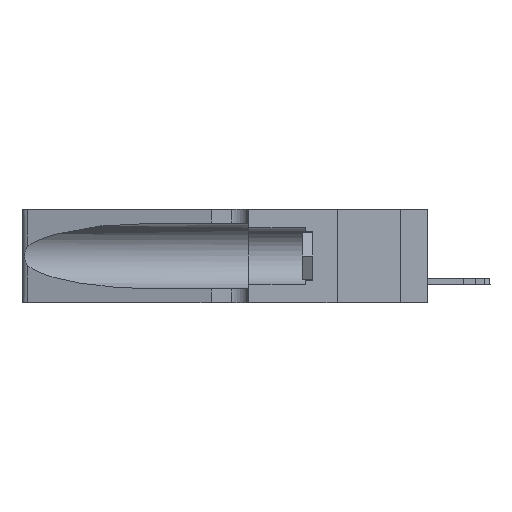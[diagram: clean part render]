
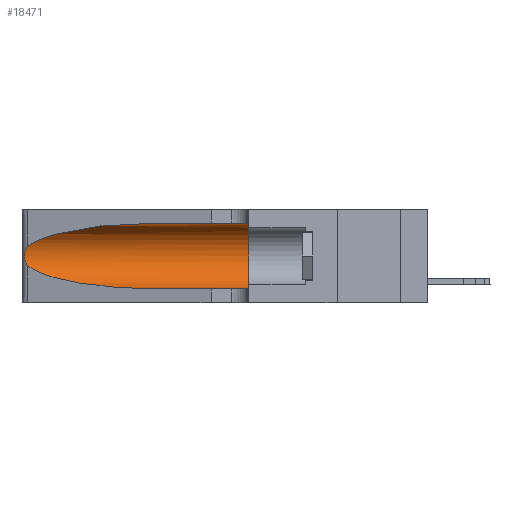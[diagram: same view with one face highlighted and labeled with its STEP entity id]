
A CAD part, left-side view. The second image highlights one B-rep face of the part: STEP entity #18471.
In plain terms, the highlighted cylindrical face has radius 3.308 mm (diameter 6.617 mm), a partial arc.
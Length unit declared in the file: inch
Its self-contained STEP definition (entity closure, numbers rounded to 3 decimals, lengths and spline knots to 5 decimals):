
#444 = CARTESIAN_POINT ( 'NONE',  ( 0.25555, 1.22993, 0.14849 ) ) ;
#629 = CARTESIAN_POINT ( 'NONE',  ( 0.25856, 1.23593, 0.16098 ) ) ;
#2391 = EDGE_CURVE ( 'NONE', #11627, #21126, #16305, .T. ) ;
#3287 = AXIS2_PLACEMENT_3D ( 'NONE', #11746, #11648, #22565 ) ;
#3627 = DIRECTION ( 'NONE',  ( 0., 1., 0. ) ) ;
#3782 = ORIENTED_EDGE ( 'NONE', *, *, #18995, .F. ) ;
#4146 = CARTESIAN_POINT ( 'NONE',  ( 0.1305, 1.61858, 0.31525 ) ) ;
#4651 = CARTESIAN_POINT ( 'NONE',  ( 0.26018, 1.23835, 0.19895 ) ) ;
#4823 = CARTESIAN_POINT ( 'NONE',  ( 0.25487, 1.22718, 0.22369 ) ) ;
#4932 = CARTESIAN_POINT ( 'NONE',  ( 0.25854, 1.2359, 0.20912 ) ) ;
#5532 = VERTEX_POINT ( 'NONE', #6572 ) ;
#6538 = CARTESIAN_POINT ( 'NONE',  ( 0.1305, 0.35, 0.05475 ) ) ;
#6572 = CARTESIAN_POINT ( 'NONE',  ( 0.1305, 0.35, 0.31525 ) ) ;
#6607 = CARTESIAN_POINT ( 'NONE',  ( 0.2373, 1.15595, 0.28018 ) ) ;
#6708 = CARTESIAN_POINT ( 'NONE',  ( 0.25639, 1.23184, 0.21858 ) ) ;
#6809 = CARTESIAN_POINT ( 'NONE',  ( 0.26075, 1.23896, 0.178 ) ) ;
#7101 = CARTESIAN_POINT ( 'NONE',  ( 0.26017, 1.23833, 0.17102 ) ) ;
#8749 = LINE ( 'NONE', #4146, #11160 ) ;
#9212 = CARTESIAN_POINT ( 'NONE',  ( 0.25487, 1.22718, 0.22369 ) ) ;
#9424 = VERTEX_POINT ( 'NONE', #26020 ) ;
#9692 = ORIENTED_EDGE ( 'NONE', *, *, #2391, .T. ) ;
#10090 = DIRECTION ( 'NONE',  ( 0., 0., 1. ) ) ;
#11160 = VECTOR ( 'NONE', #28088, 39.37008 ) ;
#11320 = CARTESIAN_POINT ( 'NONE',  ( 0.18966, 0.96281, 0.31525 ) ) ;
#11330 = CARTESIAN_POINT ( 'NONE',  ( 0.26075, 1.23896, 0.19203 ) ) ;
#11583 = CARTESIAN_POINT ( 'NONE',  ( 0.25487, 1.22718, 0.14631 ) ) ;
#11627 = VERTEX_POINT ( 'NONE', #17317 ) ;
#11648 = DIRECTION ( 'NONE',  ( 0., -1., 0. ) ) ;
#11746 = CARTESIAN_POINT ( 'NONE',  ( 0.1305, 1.61858, 0.185 ) ) ;
#11771 = CARTESIAN_POINT ( 'NONE',  ( 0.2373, 1.15595, 0.08982 ) ) ;
#12142 = VERTEX_POINT ( 'NONE', #22823 ) ;
#13289 = EDGE_LOOP ( 'NONE', ( #24638, #23947, #15255, #9692, #3782, #23756 ) ) ;
#13752 = EDGE_CURVE ( 'NONE', #9424, #12142, #21195, .T. ) ;
#13777 = CARTESIAN_POINT ( 'NONE',  ( 0.18966, 0.96281, 0.05475 ) ) ;
#14587 =( BOUNDED_CURVE ( )  B_SPLINE_CURVE ( 3, ( #11583, #11771, #13777, #18427 ),
 .UNSPECIFIED., .F., .F. ) 
 B_SPLINE_CURVE_WITH_KNOTS ( ( 4, 4 ),
 ( 3.44316, 4.71239 ),
 .UNSPECIFIED. ) 
 CURVE ( )  GEOMETRIC_REPRESENTATION_ITEM ( )  RATIONAL_B_SPLINE_CURVE ( ( 1., 0.87, 0.87, 1. ) ) 
 REPRESENTATION_ITEM ( '' )  );
#14685 = FACE_OUTER_BOUND ( 'NONE', #13289, .T. ) ;
#14928 = VECTOR ( 'NONE', #20136, 39.37008 ) ;
#15229 = CIRCLE ( 'NONE', #15394, 0.13025 ) ;
#15255 = ORIENTED_EDGE ( 'NONE', *, *, #19546, .T. ) ;
#15394 = AXIS2_PLACEMENT_3D ( 'NONE', #23144, #3627, #10090 ) ;
#16305 = LINE ( 'NONE', #24623, #14928 ) ;
#17317 = CARTESIAN_POINT ( 'NONE',  ( 0.1305, 0.72297, 0.05475 ) ) ;
#18016 = CARTESIAN_POINT ( 'NONE',  ( 0.25787, 1.23484, 0.2124 ) ) ;
#18427 = CARTESIAN_POINT ( 'NONE',  ( 0.1305, 0.72297, 0.05475 ) ) ;
#18471 = ADVANCED_FACE ( 'NONE', ( #14685 ), #21484, .F. ) ;
#18995 = EDGE_CURVE ( 'NONE', #5532, #21126, #15229, .T. ) ;
#19546 = EDGE_CURVE ( 'NONE', #12142, #11627, #14587, .T. ) ;
#19724 = CARTESIAN_POINT ( 'NONE',  ( 0.1305, 0.72297, 0.31525 ) ) ;
#20136 = DIRECTION ( 'NONE',  ( 0., -1., 0. ) ) ;
#21126 = VERTEX_POINT ( 'NONE', #6538 ) ;
#21195 = B_SPLINE_CURVE_WITH_KNOTS ( 'NONE', 3,
 ( #9212, #26789, #6708, #18016, #4932, #4651, #11330, #6809, #7101, #629, #21982, #22340, #444, #26680 ),
 .UNSPECIFIED., .F., .F.,
 ( 4, 2, 2, 2, 2, 2, 4 ),
 ( 0., 0.00027, 0.00053, 0.00107, 0.0016, 0.00187, 0.00214 ),
 .UNSPECIFIED. ) ;
#21484 = CYLINDRICAL_SURFACE ( 'NONE', #3287, 0.13025 ) ;
#21982 = CARTESIAN_POINT ( 'NONE',  ( 0.25789, 1.23486, 0.15765 ) ) ;
#22261 =( BOUNDED_CURVE ( )  B_SPLINE_CURVE ( 3, ( #19724, #11320, #6607, #4823 ),
 .UNSPECIFIED., .F., .F. ) 
 B_SPLINE_CURVE_WITH_KNOTS ( ( 4, 4 ),
 ( 1.5708, 2.84003 ),
 .UNSPECIFIED. ) 
 CURVE ( )  GEOMETRIC_REPRESENTATION_ITEM ( )  RATIONAL_B_SPLINE_CURVE ( ( 1., 0.87, 0.87, 1. ) ) 
 REPRESENTATION_ITEM ( '' )  );
#22340 = CARTESIAN_POINT ( 'NONE',  ( 0.25639, 1.23186, 0.15144 ) ) ;
#22565 = DIRECTION ( 'NONE',  ( 0., 0., -1. ) ) ;
#22823 = CARTESIAN_POINT ( 'NONE',  ( 0.25487, 1.22718, 0.14631 ) ) ;
#23144 = CARTESIAN_POINT ( 'NONE',  ( 0.1305, 0.35, 0.185 ) ) ;
#23601 = EDGE_CURVE ( 'NONE', #23856, #5532, #8749, .T. ) ;
#23756 = ORIENTED_EDGE ( 'NONE', *, *, #23601, .F. ) ;
#23856 = VERTEX_POINT ( 'NONE', #24640 ) ;
#23947 = ORIENTED_EDGE ( 'NONE', *, *, #13752, .T. ) ;
#24576 = EDGE_CURVE ( 'NONE', #23856, #9424, #22261, .T. ) ;
#24623 = CARTESIAN_POINT ( 'NONE',  ( 0.1305, 1.61858, 0.05475 ) ) ;
#24638 = ORIENTED_EDGE ( 'NONE', *, *, #24576, .T. ) ;
#24640 = CARTESIAN_POINT ( 'NONE',  ( 0.1305, 0.72297, 0.31525 ) ) ;
#26020 = CARTESIAN_POINT ( 'NONE',  ( 0.25487, 1.22718, 0.22369 ) ) ;
#26680 = CARTESIAN_POINT ( 'NONE',  ( 0.25487, 1.22718, 0.14631 ) ) ;
#26789 = CARTESIAN_POINT ( 'NONE',  ( 0.25555, 1.22994, 0.2215 ) ) ;
#28088 = DIRECTION ( 'NONE',  ( 0., -1., 0. ) ) ;
